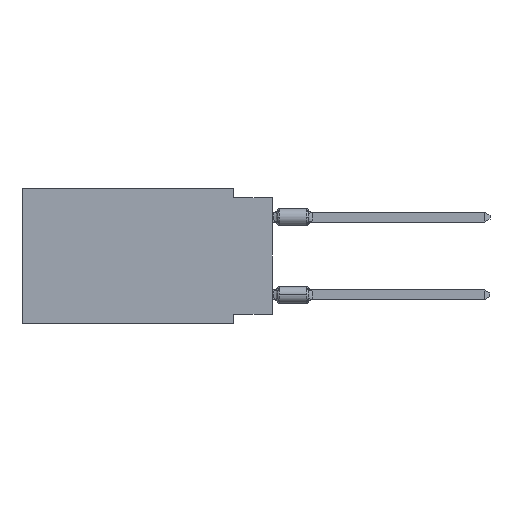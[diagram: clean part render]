
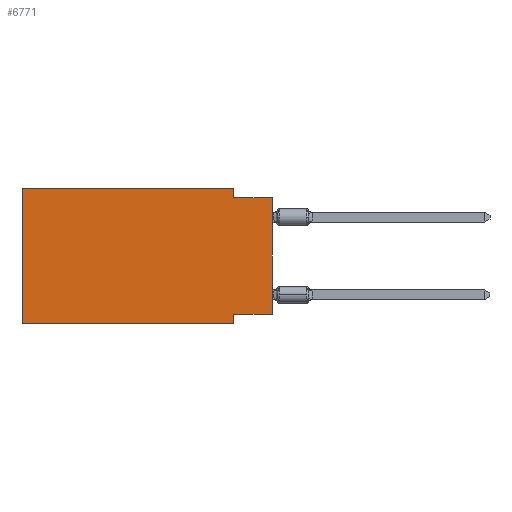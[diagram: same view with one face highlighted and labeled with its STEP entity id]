
A CAD part, left-side view. The second image highlights one B-rep face of the part: STEP entity #6771.
In plain terms, the highlighted planar face has unit normal (-1, 0, 0).
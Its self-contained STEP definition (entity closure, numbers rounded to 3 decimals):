
#208 = ORIENTED_EDGE ( 'NONE', *, *, #5612, .F. ) ;
#285 = VECTOR ( 'NONE', #11752, 1000. ) ;
#513 = CARTESIAN_POINT ( 'NONE',  ( 0., 0., -8.255 ) ) ;
#1224 = VECTOR ( 'NONE', #4190, 1000. ) ;
#1395 = DIRECTION ( 'NONE',  ( 1., 0., 0. ) ) ;
#1414 = CARTESIAN_POINT ( 'NONE',  ( 0., 2.54, -8.89 ) ) ;
#1877 = ORIENTED_EDGE ( 'NONE', *, *, #5841, .T. ) ;
#2031 = LINE ( 'NONE', #513, #13870 ) ;
#2189 = FACE_OUTER_BOUND ( 'NONE', #16597, .T. ) ;
#2482 = CARTESIAN_POINT ( 'NONE',  ( 0., 2.54, -0.635 ) ) ;
#2565 = VERTEX_POINT ( 'NONE', #3903 ) ;
#3319 = LINE ( 'NONE', #16140, #14368 ) ;
#3691 = DIRECTION ( 'NONE',  ( 0., 0., 1. ) ) ;
#3903 = CARTESIAN_POINT ( 'NONE',  ( 0., 16.383, 0. ) ) ;
#3952 = CARTESIAN_POINT ( 'NONE',  ( 0., 16.383, -8.89 ) ) ;
#4036 = LINE ( 'NONE', #3952, #15944 ) ;
#4190 = DIRECTION ( 'NONE',  ( 0., 0., 1. ) ) ;
#4195 = LINE ( 'NONE', #8207, #13254 ) ;
#4398 = VERTEX_POINT ( 'NONE', #16042 ) ;
#4534 = VECTOR ( 'NONE', #15523, 1000. ) ;
#5052 = ORIENTED_EDGE ( 'NONE', *, *, #5182, .F. ) ;
#5182 = EDGE_CURVE ( 'NONE', #7976, #13899, #2031, .T. ) ;
#5291 = LINE ( 'NONE', #8281, #1224 ) ;
#5612 = EDGE_CURVE ( 'NONE', #4398, #2565, #8643, .T. ) ;
#5653 = ORIENTED_EDGE ( 'NONE', *, *, #8578, .F. ) ;
#5841 = EDGE_CURVE ( 'NONE', #4398, #10285, #4036, .T. ) ;
#6340 = CARTESIAN_POINT ( 'NONE',  ( 0., 16.383, 0. ) ) ;
#6427 = LINE ( 'NONE', #1414, #4534 ) ;
#6771 = ADVANCED_FACE ( 'NONE', ( #2189 ), #13751, .F. ) ;
#6996 = CARTESIAN_POINT ( 'NONE',  ( 0., 0., -0.635 ) ) ;
#7185 = VERTEX_POINT ( 'NONE', #2482 ) ;
#7223 = DIRECTION ( 'NONE',  ( 0., 1., 0. ) ) ;
#7933 = ORIENTED_EDGE ( 'NONE', *, *, #15154, .F. ) ;
#7976 = VERTEX_POINT ( 'NONE', #11359 ) ;
#8037 = EDGE_CURVE ( 'NONE', #13899, #10285, #6427, .T. ) ;
#8207 = CARTESIAN_POINT ( 'NONE',  ( 0., 0., -0.635 ) ) ;
#8281 = CARTESIAN_POINT ( 'NONE',  ( 0., 0., 0. ) ) ;
#8578 = EDGE_CURVE ( 'NONE', #7185, #14557, #4195, .T. ) ;
#8643 = LINE ( 'NONE', #6340, #9432 ) ;
#8663 = DIRECTION ( 'NONE',  ( 0., -1., 0. ) ) ;
#9157 = CARTESIAN_POINT ( 'NONE',  ( 0., 2.54, 0. ) ) ;
#9211 = CARTESIAN_POINT ( 'NONE',  ( 0., 2.54, -8.255 ) ) ;
#9432 = VECTOR ( 'NONE', #3691, 1000. ) ;
#10285 = VERTEX_POINT ( 'NONE', #14603 ) ;
#10310 = LINE ( 'NONE', #12781, #285 ) ;
#10661 = DIRECTION ( 'NONE',  ( 0., -1., 0. ) ) ;
#11077 = EDGE_CURVE ( 'NONE', #7976, #14557, #5291, .T. ) ;
#11359 = CARTESIAN_POINT ( 'NONE',  ( 0., 0., -8.255 ) ) ;
#11576 = ORIENTED_EDGE ( 'NONE', *, *, #14440, .F. ) ;
#11752 = DIRECTION ( 'NONE',  ( 0., 0., -1. ) ) ;
#11836 = ORIENTED_EDGE ( 'NONE', *, *, #11077, .T. ) ;
#12554 = DIRECTION ( 'NONE',  ( 0., 0., -1. ) ) ;
#12781 = CARTESIAN_POINT ( 'NONE',  ( 0., 2.54, 0. ) ) ;
#13043 = CARTESIAN_POINT ( 'NONE',  ( 0., 16.383, 0. ) ) ;
#13254 = VECTOR ( 'NONE', #10661, 1000. ) ;
#13664 = VERTEX_POINT ( 'NONE', #9157 ) ;
#13751 = PLANE ( 'NONE',  #16724 ) ;
#13870 = VECTOR ( 'NONE', #7223, 1000. ) ;
#13899 = VERTEX_POINT ( 'NONE', #9211 ) ;
#13914 = ORIENTED_EDGE ( 'NONE', *, *, #8037, .F. ) ;
#14368 = VECTOR ( 'NONE', #8663, 1000. ) ;
#14440 = EDGE_CURVE ( 'NONE', #13664, #7185, #10310, .T. ) ;
#14494 = DIRECTION ( 'NONE',  ( 0., -1., 0. ) ) ;
#14557 = VERTEX_POINT ( 'NONE', #6996 ) ;
#14603 = CARTESIAN_POINT ( 'NONE',  ( 0., 2.54, -8.89 ) ) ;
#15154 = EDGE_CURVE ( 'NONE', #2565, #13664, #3319, .T. ) ;
#15523 = DIRECTION ( 'NONE',  ( 0., 0., -1. ) ) ;
#15944 = VECTOR ( 'NONE', #14494, 1000. ) ;
#16042 = CARTESIAN_POINT ( 'NONE',  ( 0., 16.383, -8.89 ) ) ;
#16140 = CARTESIAN_POINT ( 'NONE',  ( 0., 16.383, 0. ) ) ;
#16597 = EDGE_LOOP ( 'NONE', ( #11836, #5653, #11576, #7933, #208, #1877, #13914, #5052 ) ) ;
#16724 = AXIS2_PLACEMENT_3D ( 'NONE', #13043, #1395, #12554 ) ;
